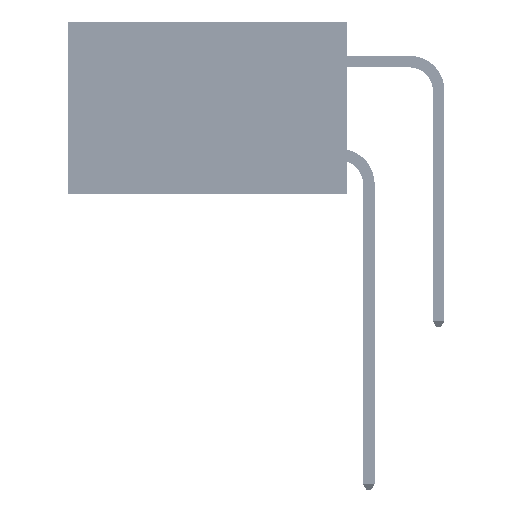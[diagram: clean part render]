
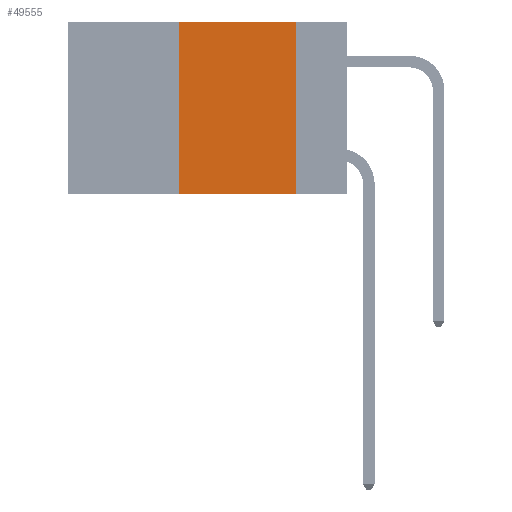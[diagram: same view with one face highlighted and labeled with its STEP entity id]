
A CAD part, left-side view. The second image highlights one B-rep face of the part: STEP entity #49555.
In plain terms, the highlighted planar face has unit normal (-1, 0, 0).
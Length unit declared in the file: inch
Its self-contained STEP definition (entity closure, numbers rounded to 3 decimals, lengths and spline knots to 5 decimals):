
#4006 = EDGE_CURVE ( 'NONE', #36318, #22452, #33599, .T. ) ;
#5488 = ORIENTED_EDGE ( 'NONE', *, *, #6664, .F. ) ;
#5850 = PLANE ( 'NONE',  #12845 ) ;
#6259 = CARTESIAN_POINT ( 'NONE',  ( 0., 0.6, 0. ) ) ;
#6664 = EDGE_CURVE ( 'NONE', #36318, #51399, #28134, .T. ) ;
#10710 = CARTESIAN_POINT ( 'NONE',  ( 0., 0.11, -0.37 ) ) ;
#11161 = VECTOR ( 'NONE', #49514, 39.37008 ) ;
#12781 = DIRECTION ( 'NONE',  ( 0., 0., -1. ) ) ;
#12845 = AXIS2_PLACEMENT_3D ( 'NONE', #39490, #14486, #27381 ) ;
#13247 = EDGE_LOOP ( 'NONE', ( #53395, #40086, #5488, #42425 ) ) ;
#13412 = CARTESIAN_POINT ( 'NONE',  ( 0., 0.36, 0. ) ) ;
#13550 = VECTOR ( 'NONE', #12781, 39.37008 ) ;
#14486 = DIRECTION ( 'NONE',  ( 1., 0., 0. ) ) ;
#16400 = EDGE_CURVE ( 'NONE', #51399, #43517, #24063, .T. ) ;
#18053 = DIRECTION ( 'NONE',  ( 0., 0., 1. ) ) ;
#22452 = VERTEX_POINT ( 'NONE', #10710 ) ;
#23913 = EDGE_CURVE ( 'NONE', #43517, #22452, #52284, .T. ) ;
#24063 = LINE ( 'NONE', #6259, #50262 ) ;
#25569 = CARTESIAN_POINT ( 'NONE',  ( 0., 0.11, 0. ) ) ;
#27381 = DIRECTION ( 'NONE',  ( 0., 0., -1. ) ) ;
#28134 = LINE ( 'NONE', #13412, #48383 ) ;
#28682 = CARTESIAN_POINT ( 'NONE',  ( 0., 0.11, 0. ) ) ;
#33599 = LINE ( 'NONE', #45695, #11161 ) ;
#36318 = VERTEX_POINT ( 'NONE', #50960 ) ;
#39490 = CARTESIAN_POINT ( 'NONE',  ( 0., 0.6, 0. ) ) ;
#40086 = ORIENTED_EDGE ( 'NONE', *, *, #16400, .F. ) ;
#42425 = ORIENTED_EDGE ( 'NONE', *, *, #4006, .T. ) ;
#43517 = VERTEX_POINT ( 'NONE', #25569 ) ;
#43933 = FACE_OUTER_BOUND ( 'NONE', #13247, .T. ) ;
#45695 = CARTESIAN_POINT ( 'NONE',  ( 0., 0.6, -0.37 ) ) ;
#48383 = VECTOR ( 'NONE', #18053, 39.37008 ) ;
#49514 = DIRECTION ( 'NONE',  ( 0., -1., 0. ) ) ;
#49555 = ADVANCED_FACE ( 'NONE', ( #43933 ), #5850, .F. ) ;
#50262 = VECTOR ( 'NONE', #51568, 39.37008 ) ;
#50960 = CARTESIAN_POINT ( 'NONE',  ( 0., 0.36, -0.37 ) ) ;
#51399 = VERTEX_POINT ( 'NONE', #52758 ) ;
#51568 = DIRECTION ( 'NONE',  ( 0., -1., 0. ) ) ;
#52284 = LINE ( 'NONE', #28682, #13550 ) ;
#52758 = CARTESIAN_POINT ( 'NONE',  ( 0., 0.36, 0. ) ) ;
#53395 = ORIENTED_EDGE ( 'NONE', *, *, #23913, .F. ) ;
